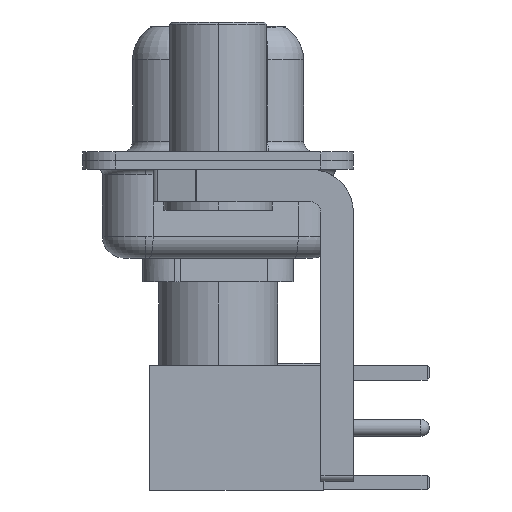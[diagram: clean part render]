
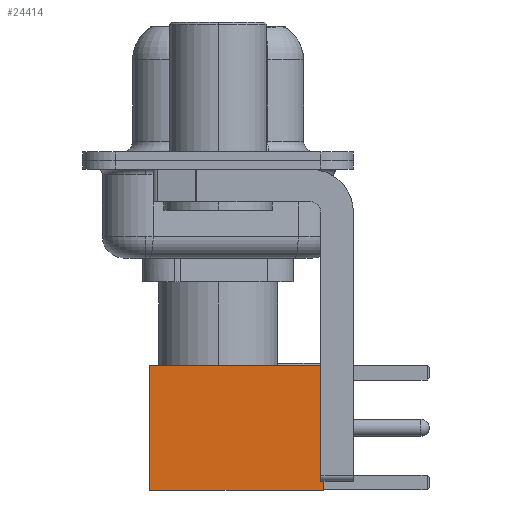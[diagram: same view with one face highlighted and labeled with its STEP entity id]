
A CAD part, left-side view. The second image highlights one B-rep face of the part: STEP entity #24414.
In plain terms, the highlighted face is planar.
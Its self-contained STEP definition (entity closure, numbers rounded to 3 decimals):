
#457 = CARTESIAN_POINT ( 'NONE',  ( 0., 2.875, 8. ) ) ;
#513 = CARTESIAN_POINT ( 'NONE',  ( -2.875, 2.875, 0. ) ) ;
#650 = DIRECTION ( 'NONE',  ( 0., 0., 1. ) ) ;
#950 = DIRECTION ( 'NONE',  ( 0., 1., 0. ) ) ;
#2189 = VECTOR ( 'NONE', #10650, 1000. ) ;
#2363 = CARTESIAN_POINT ( 'NONE',  ( -2.875, 2.875, 8. ) ) ;
#2968 = LINE ( 'NONE', #19364, #13190 ) ;
#3081 = CARTESIAN_POINT ( 'NONE',  ( 2.875, 2.875, 0. ) ) ;
#4863 = CARTESIAN_POINT ( 'NONE',  ( 0., 2.875, 0. ) ) ;
#5199 = EDGE_CURVE ( 'NONE', #23403, #10222, #23079, .T. ) ;
#5455 = DIRECTION ( 'NONE',  ( -1., 0., 0. ) ) ;
#5504 = PLANE ( 'NONE',  #9888 ) ;
#6460 = ORIENTED_EDGE ( 'NONE', *, *, #17515, .T. ) ;
#6736 = CARTESIAN_POINT ( 'NONE',  ( 2.875, 2.875, 0. ) ) ;
#7815 = DIRECTION ( 'NONE',  ( 0., 0., -1. ) ) ;
#8622 = ORIENTED_EDGE ( 'NONE', *, *, #27428, .F. ) ;
#8977 = DIRECTION ( 'NONE',  ( -1., 0., 0. ) ) ;
#9878 = LINE ( 'NONE', #457, #11095 ) ;
#9888 = AXIS2_PLACEMENT_3D ( 'NONE', #3081, #950, #650 ) ;
#10222 = VERTEX_POINT ( 'NONE', #513 ) ;
#10650 = DIRECTION ( 'NONE',  ( 0., 0., -1. ) ) ;
#11095 = VECTOR ( 'NONE', #5455, 1000. ) ;
#12298 = VERTEX_POINT ( 'NONE', #25093 ) ;
#13190 = VECTOR ( 'NONE', #7815, 1000. ) ;
#15566 = EDGE_CURVE ( 'NONE', #12298, #20593, #9878, .T. ) ;
#16342 = ORIENTED_EDGE ( 'NONE', *, *, #5199, .T. ) ;
#16689 = VECTOR ( 'NONE', #8977, 1000. ) ;
#17515 = EDGE_CURVE ( 'NONE', #12298, #23403, #2968, .T. ) ;
#19364 = CARTESIAN_POINT ( 'NONE',  ( 2.875, 2.875, 0. ) ) ;
#20593 = VERTEX_POINT ( 'NONE', #2363 ) ;
#23079 = LINE ( 'NONE', #4863, #16689 ) ;
#23403 = VERTEX_POINT ( 'NONE', #6736 ) ;
#23444 = FACE_OUTER_BOUND ( 'NONE', #25564, .T. ) ;
#24414 = ADVANCED_FACE ( 'NONE', ( #23444 ), #5504, .T. ) ;
#24476 = CARTESIAN_POINT ( 'NONE',  ( -2.875, 2.875, 0. ) ) ;
#25093 = CARTESIAN_POINT ( 'NONE',  ( 2.875, 2.875, 8. ) ) ;
#25564 = EDGE_LOOP ( 'NONE', ( #6460, #16342, #8622, #29654 ) ) ;
#27428 = EDGE_CURVE ( 'NONE', #20593, #10222, #29475, .T. ) ;
#29475 = LINE ( 'NONE', #24476, #2189 ) ;
#29654 = ORIENTED_EDGE ( 'NONE', *, *, #15566, .F. ) ;
